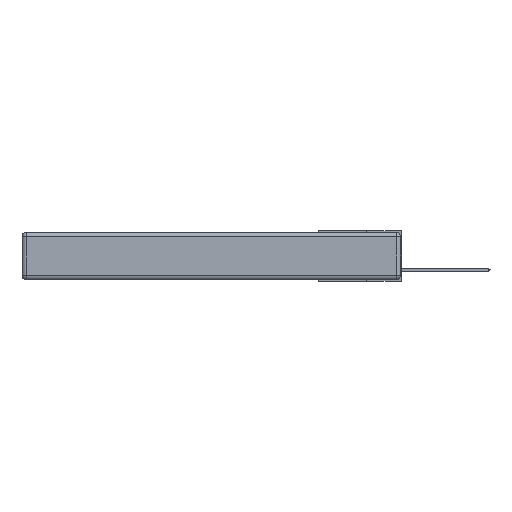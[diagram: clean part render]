
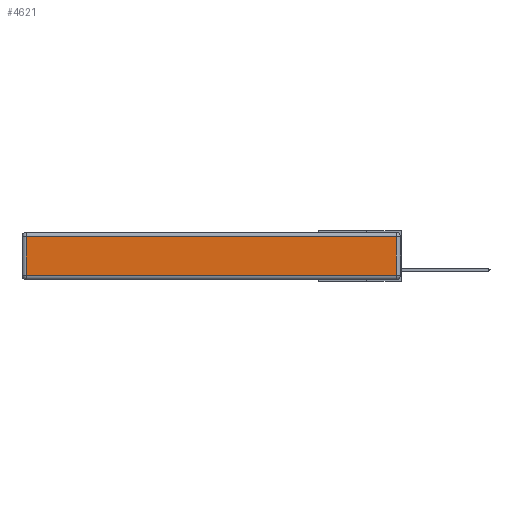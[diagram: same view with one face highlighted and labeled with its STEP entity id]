
A CAD part, left-side view. The second image highlights one B-rep face of the part: STEP entity #4621.
In plain terms, the highlighted planar face has unit normal (-1, 0, 0).
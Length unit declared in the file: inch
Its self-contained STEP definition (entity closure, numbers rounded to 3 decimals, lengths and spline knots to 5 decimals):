
#378 = PLANE ( 'NONE',  #3360 ) ;
#425 = CARTESIAN_POINT ( 'NONE',  ( 0., 0.03, -0.343 ) ) ;
#1098 = FACE_OUTER_BOUND ( 'NONE', #17352, .T. ) ;
#3033 = VERTEX_POINT ( 'NONE', #25517 ) ;
#3360 = AXIS2_PLACEMENT_3D ( 'NONE', #21099, #12925, #21196 ) ;
#4621 = ADVANCED_FACE ( 'NONE', ( #1098 ), #378, .T. ) ;
#5583 = EDGE_CURVE ( 'NONE', #6954, #17047, #19147, .T. ) ;
#5623 = ORIENTED_EDGE ( 'NONE', *, *, #5583, .T. ) ;
#5970 = VECTOR ( 'NONE', #21241, 39.37008 ) ;
#6750 = EDGE_CURVE ( 'NONE', #24069, #3033, #11558, .T. ) ;
#6954 = VERTEX_POINT ( 'NONE', #11920 ) ;
#7294 = CARTESIAN_POINT ( 'NONE',  ( 0., 2.72, -0.313 ) ) ;
#7565 = VECTOR ( 'NONE', #14140, 39.37008 ) ;
#7890 = EDGE_CURVE ( 'NONE', #3033, #6954, #8535, .T. ) ;
#8535 = LINE ( 'NONE', #10455, #19680 ) ;
#8548 = CARTESIAN_POINT ( 'NONE',  ( 0., 2.72, -0.343 ) ) ;
#9934 = VECTOR ( 'NONE', #16714, 39.37008 ) ;
#10455 = CARTESIAN_POINT ( 'NONE',  ( 0., 2.75, -0.03 ) ) ;
#11558 = LINE ( 'NONE', #425, #5970 ) ;
#11830 = ORIENTED_EDGE ( 'NONE', *, *, #6750, .T. ) ;
#11920 = CARTESIAN_POINT ( 'NONE',  ( 0., 2.72, -0.03 ) ) ;
#12925 = DIRECTION ( 'NONE',  ( -1., 0., 0. ) ) ;
#13204 = LINE ( 'NONE', #24266, #7565 ) ;
#14140 = DIRECTION ( 'NONE',  ( 0., -1., 0. ) ) ;
#14894 = DIRECTION ( 'NONE',  ( 0., 1., 0. ) ) ;
#16402 = ORIENTED_EDGE ( 'NONE', *, *, #18759, .T. ) ;
#16714 = DIRECTION ( 'NONE',  ( 0., 0., -1. ) ) ;
#17047 = VERTEX_POINT ( 'NONE', #7294 ) ;
#17352 = EDGE_LOOP ( 'NONE', ( #16402, #11830, #19683, #5623 ) ) ;
#18759 = EDGE_CURVE ( 'NONE', #17047, #24069, #13204, .T. ) ;
#19147 = LINE ( 'NONE', #8548, #9934 ) ;
#19680 = VECTOR ( 'NONE', #14894, 39.37008 ) ;
#19683 = ORIENTED_EDGE ( 'NONE', *, *, #7890, .T. ) ;
#21099 = CARTESIAN_POINT ( 'NONE',  ( 0., 0., -0.343 ) ) ;
#21196 = DIRECTION ( 'NONE',  ( 0., 0., 1. ) ) ;
#21241 = DIRECTION ( 'NONE',  ( 0., 0., 1. ) ) ;
#24069 = VERTEX_POINT ( 'NONE', #25299 ) ;
#24266 = CARTESIAN_POINT ( 'NONE',  ( 0., 0., -0.313 ) ) ;
#25299 = CARTESIAN_POINT ( 'NONE',  ( 0., 0.03, -0.313 ) ) ;
#25517 = CARTESIAN_POINT ( 'NONE',  ( 0., 0.03, -0.03 ) ) ;
